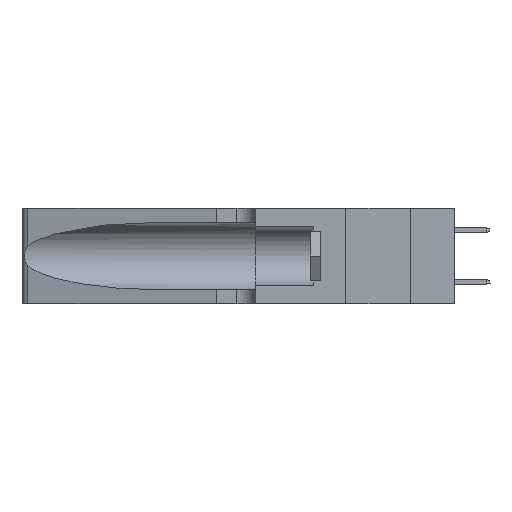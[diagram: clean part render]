
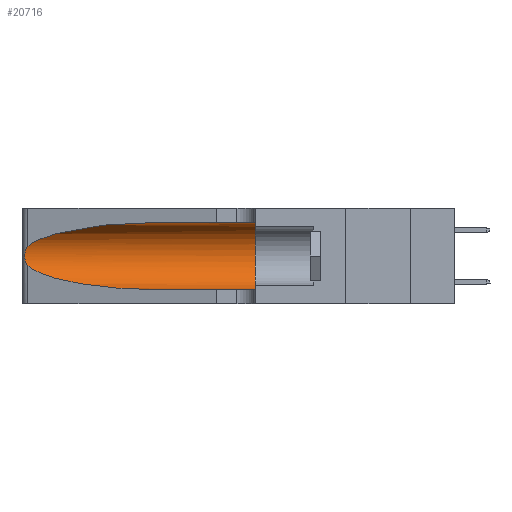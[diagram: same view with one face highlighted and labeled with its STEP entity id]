
A CAD part, left-side view. The second image highlights one B-rep face of the part: STEP entity #20716.
In plain terms, the highlighted cylindrical face has radius 3.308 mm (diameter 6.617 mm), a partial arc.
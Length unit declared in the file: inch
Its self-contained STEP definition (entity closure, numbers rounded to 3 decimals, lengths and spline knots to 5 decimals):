
#604 = EDGE_CURVE ( 'NONE', #6900, #4813, #12686, .T. ) ;
#1225 = VERTEX_POINT ( 'NONE', #23627 ) ;
#1439 = B_SPLINE_CURVE_WITH_KNOTS ( 'NONE', 3,
 ( #7300, #15831, #16105, #26687, #24338, #11885, #11615, #24744, #24605, #9257, #9524, #13999, #3389, #20418 ),
 .UNSPECIFIED., .F., .F.,
 ( 4, 2, 2, 2, 2, 2, 4 ),
 ( 0., 0.00027, 0.00053, 0.00107, 0.0016, 0.00187, 0.00214 ),
 .UNSPECIFIED. ) ;
#3330 = DIRECTION ( 'NONE',  ( 0., 0., 1. ) ) ;
#3389 = CARTESIAN_POINT ( 'NONE',  ( 0.25555, 1.22993, 0.14849 ) ) ;
#3698 = VECTOR ( 'NONE', #9019, 39.37008 ) ;
#4813 = VERTEX_POINT ( 'NONE', #16010 ) ;
#4815 = DIRECTION ( 'NONE',  ( 0., -1., 0. ) ) ;
#5682 = DIRECTION ( 'NONE',  ( 0., -1., 0. ) ) ;
#5713 = EDGE_CURVE ( 'NONE', #11032, #1225, #21091, .T. ) ;
#6529 = CARTESIAN_POINT ( 'NONE',  ( 0.2373, 1.15595, 0.08982 ) ) ;
#6900 = VERTEX_POINT ( 'NONE', #26449 ) ;
#7210 = VECTOR ( 'NONE', #4815, 39.37008 ) ;
#7300 = CARTESIAN_POINT ( 'NONE',  ( 0.25487, 1.22718, 0.22369 ) ) ;
#7769 = CYLINDRICAL_SURFACE ( 'NONE', #8339, 0.13025 ) ;
#8339 = AXIS2_PLACEMENT_3D ( 'NONE', #9997, #5682, #15805 ) ;
#9019 = DIRECTION ( 'NONE',  ( 0., -1., 0. ) ) ;
#9257 = CARTESIAN_POINT ( 'NONE',  ( 0.25856, 1.23593, 0.16098 ) ) ;
#9524 = CARTESIAN_POINT ( 'NONE',  ( 0.25789, 1.23486, 0.15765 ) ) ;
#9569 = LINE ( 'NONE', #22288, #3698 ) ;
#9678 = CARTESIAN_POINT ( 'NONE',  ( 0.18966, 0.96281, 0.31525 ) ) ;
#9893 = EDGE_CURVE ( 'NONE', #4813, #16053, #15147, .T. ) ;
#9997 = CARTESIAN_POINT ( 'NONE',  ( 0.1305, 1.61858, 0.185 ) ) ;
#10206 = CARTESIAN_POINT ( 'NONE',  ( 0.1305, 0.35, 0.05475 ) ) ;
#11032 = VERTEX_POINT ( 'NONE', #24430 ) ;
#11615 = CARTESIAN_POINT ( 'NONE',  ( 0.26075, 1.23896, 0.19203 ) ) ;
#11885 = CARTESIAN_POINT ( 'NONE',  ( 0.26018, 1.23835, 0.19895 ) ) ;
#12484 = AXIS2_PLACEMENT_3D ( 'NONE', #20488, #18262, #3330 ) ;
#12528 = ORIENTED_EDGE ( 'NONE', *, *, #5713, .T. ) ;
#12686 =( BOUNDED_CURVE ( )  B_SPLINE_CURVE ( 3, ( #15333, #6529, #17429, #25941 ),
 .UNSPECIFIED., .F., .T. ) 
 B_SPLINE_CURVE_WITH_KNOTS ( ( 4, 4 ),
 ( 3.44316, 4.71239 ),
 .UNSPECIFIED. ) 
 CURVE ( )  GEOMETRIC_REPRESENTATION_ITEM ( )  RATIONAL_B_SPLINE_CURVE ( ( 1., 0.87, 0.87, 1. ) ) 
 REPRESENTATION_ITEM ( '' )  );
#13609 = EDGE_CURVE ( 'NONE', #1225, #6900, #1439, .T. ) ;
#13999 = CARTESIAN_POINT ( 'NONE',  ( 0.25639, 1.23186, 0.15144 ) ) ;
#14104 = EDGE_CURVE ( 'NONE', #11032, #22470, #9569, .T. ) ;
#15147 = LINE ( 'NONE', #23667, #7210 ) ;
#15333 = CARTESIAN_POINT ( 'NONE',  ( 0.25487, 1.22718, 0.14631 ) ) ;
#15683 = ORIENTED_EDGE ( 'NONE', *, *, #14104, .F. ) ;
#15805 = DIRECTION ( 'NONE',  ( 0., 0., -1. ) ) ;
#15831 = CARTESIAN_POINT ( 'NONE',  ( 0.25555, 1.22994, 0.2215 ) ) ;
#16010 = CARTESIAN_POINT ( 'NONE',  ( 0.1305, 0.72297, 0.05475 ) ) ;
#16053 = VERTEX_POINT ( 'NONE', #10206 ) ;
#16105 = CARTESIAN_POINT ( 'NONE',  ( 0.25639, 1.23184, 0.21858 ) ) ;
#16128 = CARTESIAN_POINT ( 'NONE',  ( 0.25487, 1.22718, 0.22369 ) ) ;
#16216 = ORIENTED_EDGE ( 'NONE', *, *, #604, .T. ) ;
#16402 = CARTESIAN_POINT ( 'NONE',  ( 0.2373, 1.15595, 0.28018 ) ) ;
#17429 = CARTESIAN_POINT ( 'NONE',  ( 0.18966, 0.96281, 0.05475 ) ) ;
#17606 = FACE_OUTER_BOUND ( 'NONE', #21635, .T. ) ;
#18262 = DIRECTION ( 'NONE',  ( 0., 1., 0. ) ) ;
#19807 = CARTESIAN_POINT ( 'NONE',  ( 0.1305, 0.35, 0.31525 ) ) ;
#20418 = CARTESIAN_POINT ( 'NONE',  ( 0.25487, 1.22718, 0.14631 ) ) ;
#20488 = CARTESIAN_POINT ( 'NONE',  ( 0.1305, 0.35, 0.185 ) ) ;
#20716 = ADVANCED_FACE ( 'NONE', ( #17606 ), #7769, .F. ) ;
#20967 = CIRCLE ( 'NONE', #12484, 0.13025 ) ;
#21091 =( BOUNDED_CURVE ( )  B_SPLINE_CURVE ( 3, ( #24497, #9678, #16402, #16128 ),
 .UNSPECIFIED., .F., .T. ) 
 B_SPLINE_CURVE_WITH_KNOTS ( ( 4, 4 ),
 ( 1.5708, 2.84003 ),
 .UNSPECIFIED. ) 
 CURVE ( )  GEOMETRIC_REPRESENTATION_ITEM ( )  RATIONAL_B_SPLINE_CURVE ( ( 1., 0.87, 0.87, 1. ) ) 
 REPRESENTATION_ITEM ( '' )  );
#21635 = EDGE_LOOP ( 'NONE', ( #12528, #25728, #16216, #22795, #26139, #15683 ) ) ;
#22288 = CARTESIAN_POINT ( 'NONE',  ( 0.1305, 1.61858, 0.31525 ) ) ;
#22470 = VERTEX_POINT ( 'NONE', #19807 ) ;
#22795 = ORIENTED_EDGE ( 'NONE', *, *, #9893, .T. ) ;
#23627 = CARTESIAN_POINT ( 'NONE',  ( 0.25487, 1.22718, 0.22369 ) ) ;
#23667 = CARTESIAN_POINT ( 'NONE',  ( 0.1305, 1.61858, 0.05475 ) ) ;
#24338 = CARTESIAN_POINT ( 'NONE',  ( 0.25854, 1.2359, 0.20912 ) ) ;
#24430 = CARTESIAN_POINT ( 'NONE',  ( 0.1305, 0.72297, 0.31525 ) ) ;
#24497 = CARTESIAN_POINT ( 'NONE',  ( 0.1305, 0.72297, 0.31525 ) ) ;
#24605 = CARTESIAN_POINT ( 'NONE',  ( 0.26017, 1.23833, 0.17102 ) ) ;
#24744 = CARTESIAN_POINT ( 'NONE',  ( 0.26075, 1.23896, 0.178 ) ) ;
#25728 = ORIENTED_EDGE ( 'NONE', *, *, #13609, .T. ) ;
#25861 = EDGE_CURVE ( 'NONE', #22470, #16053, #20967, .T. ) ;
#25941 = CARTESIAN_POINT ( 'NONE',  ( 0.1305, 0.72297, 0.05475 ) ) ;
#26139 = ORIENTED_EDGE ( 'NONE', *, *, #25861, .F. ) ;
#26449 = CARTESIAN_POINT ( 'NONE',  ( 0.25487, 1.22718, 0.14631 ) ) ;
#26687 = CARTESIAN_POINT ( 'NONE',  ( 0.25787, 1.23484, 0.2124 ) ) ;
